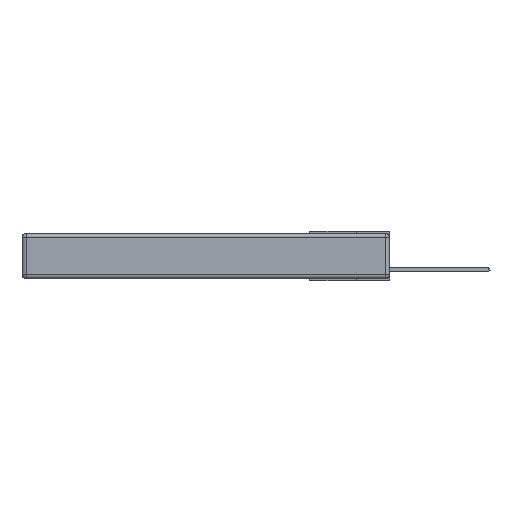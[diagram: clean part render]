
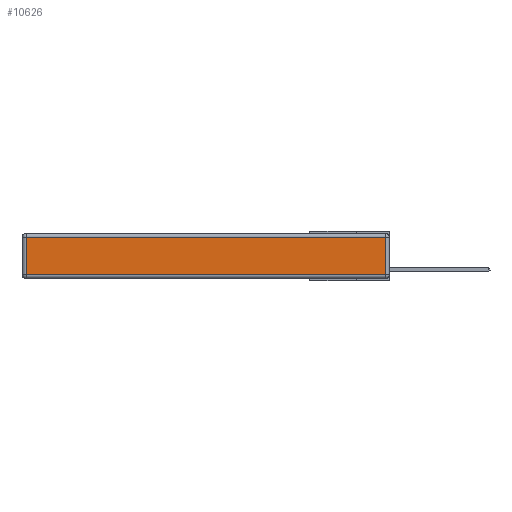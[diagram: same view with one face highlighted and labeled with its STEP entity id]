
A CAD part, left-side view. The second image highlights one B-rep face of the part: STEP entity #10626.
In plain terms, the highlighted planar face has unit normal (-1, 0, 0).
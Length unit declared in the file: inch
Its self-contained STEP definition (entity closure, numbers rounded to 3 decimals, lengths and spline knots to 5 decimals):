
#971 = ORIENTED_EDGE ( 'NONE', *, *, #1705, .T. ) ;
#1294 = EDGE_CURVE ( 'NONE', #15610, #16638, #12207, .T. ) ;
#1454 = CARTESIAN_POINT ( 'NONE',  ( 0., 2.72, -0.03 ) ) ;
#1705 = EDGE_CURVE ( 'NONE', #11732, #23204, #12512, .T. ) ;
#3167 = PLANE ( 'NONE',  #23063 ) ;
#3448 = VECTOR ( 'NONE', #17894, 39.37008 ) ;
#4937 = DIRECTION ( 'NONE',  ( 0., 0., -1. ) ) ;
#4988 = CARTESIAN_POINT ( 'NONE',  ( 0., 0., -0.343 ) ) ;
#5201 = CARTESIAN_POINT ( 'NONE',  ( 0., 0.03, -0.03 ) ) ;
#5891 = VECTOR ( 'NONE', #7139, 39.37008 ) ;
#6071 = EDGE_LOOP ( 'NONE', ( #10682, #971, #11069, #6596 ) ) ;
#6522 = FACE_OUTER_BOUND ( 'NONE', #6071, .T. ) ;
#6596 = ORIENTED_EDGE ( 'NONE', *, *, #1294, .T. ) ;
#7139 = DIRECTION ( 'NONE',  ( 0., -1., 0. ) ) ;
#7857 = EDGE_CURVE ( 'NONE', #23204, #15610, #11980, .T. ) ;
#8178 = CARTESIAN_POINT ( 'NONE',  ( 0., 2.75, -0.03 ) ) ;
#8889 = CARTESIAN_POINT ( 'NONE',  ( 0., 0., -0.313 ) ) ;
#9083 = VECTOR ( 'NONE', #4937, 39.37008 ) ;
#10082 = DIRECTION ( 'NONE',  ( 0., 1., 0. ) ) ;
#10626 = ADVANCED_FACE ( 'NONE', ( #6522 ), #3167, .T. ) ;
#10682 = ORIENTED_EDGE ( 'NONE', *, *, #14949, .T. ) ;
#11069 = ORIENTED_EDGE ( 'NONE', *, *, #7857, .T. ) ;
#11732 = VERTEX_POINT ( 'NONE', #20586 ) ;
#11980 = LINE ( 'NONE', #8178, #22000 ) ;
#12207 = LINE ( 'NONE', #14923, #9083 ) ;
#12467 = LINE ( 'NONE', #8889, #5891 ) ;
#12512 = LINE ( 'NONE', #14127, #3448 ) ;
#13045 = DIRECTION ( 'NONE',  ( -1., 0., 0. ) ) ;
#14127 = CARTESIAN_POINT ( 'NONE',  ( 0., 0.03, -0.343 ) ) ;
#14923 = CARTESIAN_POINT ( 'NONE',  ( 0., 2.72, -0.343 ) ) ;
#14949 = EDGE_CURVE ( 'NONE', #16638, #11732, #12467, .T. ) ;
#15610 = VERTEX_POINT ( 'NONE', #1454 ) ;
#16638 = VERTEX_POINT ( 'NONE', #22362 ) ;
#17894 = DIRECTION ( 'NONE',  ( 0., 0., 1. ) ) ;
#20586 = CARTESIAN_POINT ( 'NONE',  ( 0., 0.03, -0.313 ) ) ;
#22000 = VECTOR ( 'NONE', #10082, 39.37008 ) ;
#22362 = CARTESIAN_POINT ( 'NONE',  ( 0., 2.72, -0.313 ) ) ;
#23063 = AXIS2_PLACEMENT_3D ( 'NONE', #4988, #13045, #24982 ) ;
#23204 = VERTEX_POINT ( 'NONE', #5201 ) ;
#24982 = DIRECTION ( 'NONE',  ( 0., 0., 1. ) ) ;
